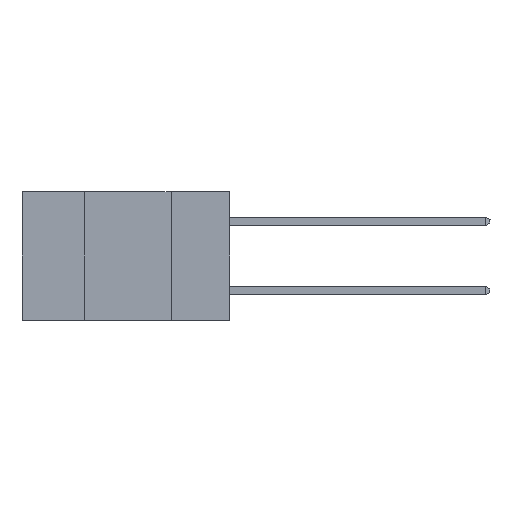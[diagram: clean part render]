
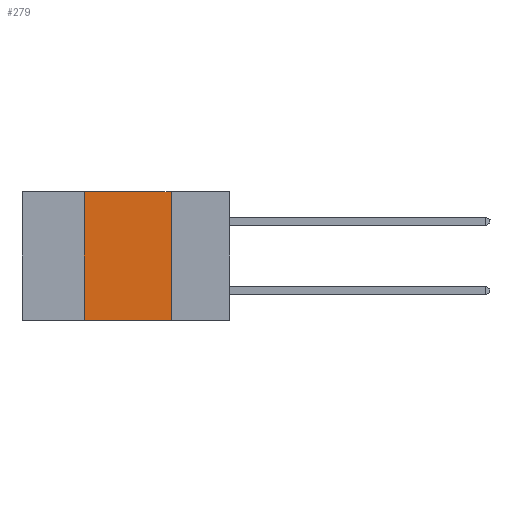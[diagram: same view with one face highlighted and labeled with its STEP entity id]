
A CAD part, left-side view. The second image highlights one B-rep face of the part: STEP entity #279.
In plain terms, the highlighted planar face has unit normal (-1, 0, 0).
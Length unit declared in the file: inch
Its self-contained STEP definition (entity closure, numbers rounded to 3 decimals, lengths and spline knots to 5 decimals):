
#5 = CARTESIAN_POINT ( 'NONE',  ( 0., 0.17, -0.37 ) ) ;
#275 = LINE ( 'NONE', #7927, #2352 ) ;
#279 = ADVANCED_FACE ( 'NONE', ( #5422 ), #895, .F. ) ;
#769 = DIRECTION ( 'NONE',  ( 0., 0., -1. ) ) ;
#843 = VECTOR ( 'NONE', #5528, 39.37008 ) ;
#895 = PLANE ( 'NONE',  #4392 ) ;
#1375 = LINE ( 'NONE', #5173, #1873 ) ;
#1460 = CARTESIAN_POINT ( 'NONE',  ( 0., 0.42, -0.37 ) ) ;
#1596 = DIRECTION ( 'NONE',  ( 0., 0., 1. ) ) ;
#1873 = VECTOR ( 'NONE', #8988, 39.37008 ) ;
#2352 = VECTOR ( 'NONE', #10772, 39.37008 ) ;
#2386 = VERTEX_POINT ( 'NONE', #5912 ) ;
#2675 = DIRECTION ( 'NONE',  ( 1., 0., 0. ) ) ;
#2771 = ORIENTED_EDGE ( 'NONE', *, *, #5413, .T. ) ;
#4016 = LINE ( 'NONE', #8280, #843 ) ;
#4392 = AXIS2_PLACEMENT_3D ( 'NONE', #12208, #2675, #769 ) ;
#4551 = CARTESIAN_POINT ( 'NONE',  ( 0., 0.42, 0. ) ) ;
#4739 = VERTEX_POINT ( 'NONE', #4551 ) ;
#5173 = CARTESIAN_POINT ( 'NONE',  ( 0., 0.17, -0.37 ) ) ;
#5413 = EDGE_CURVE ( 'NONE', #11435, #9560, #275, .T. ) ;
#5422 = FACE_OUTER_BOUND ( 'NONE', #10182, .T. ) ;
#5528 = DIRECTION ( 'NONE',  ( 0., -1., 0. ) ) ;
#5912 = CARTESIAN_POINT ( 'NONE',  ( 0., 0.17, 0. ) ) ;
#6273 = LINE ( 'NONE', #1460, #11951 ) ;
#6523 = ORIENTED_EDGE ( 'NONE', *, *, #7810, .F. ) ;
#7694 = EDGE_CURVE ( 'NONE', #4739, #2386, #4016, .T. ) ;
#7810 = EDGE_CURVE ( 'NONE', #11435, #4739, #6273, .T. ) ;
#7927 = CARTESIAN_POINT ( 'NONE',  ( 0., 0.6, -0.37 ) ) ;
#8280 = CARTESIAN_POINT ( 'NONE',  ( 0., 0.6, 0. ) ) ;
#8988 = DIRECTION ( 'NONE',  ( 0., 0., -1. ) ) ;
#9103 = CARTESIAN_POINT ( 'NONE',  ( 0., 0.42, -0.37 ) ) ;
#9560 = VERTEX_POINT ( 'NONE', #5 ) ;
#9811 = ORIENTED_EDGE ( 'NONE', *, *, #7694, .F. ) ;
#10182 = EDGE_LOOP ( 'NONE', ( #12076, #9811, #6523, #2771 ) ) ;
#10772 = DIRECTION ( 'NONE',  ( 0., -1., 0. ) ) ;
#11133 = EDGE_CURVE ( 'NONE', #2386, #9560, #1375, .T. ) ;
#11435 = VERTEX_POINT ( 'NONE', #9103 ) ;
#11951 = VECTOR ( 'NONE', #1596, 39.37008 ) ;
#12076 = ORIENTED_EDGE ( 'NONE', *, *, #11133, .F. ) ;
#12208 = CARTESIAN_POINT ( 'NONE',  ( 0., 0.6, 0. ) ) ;
